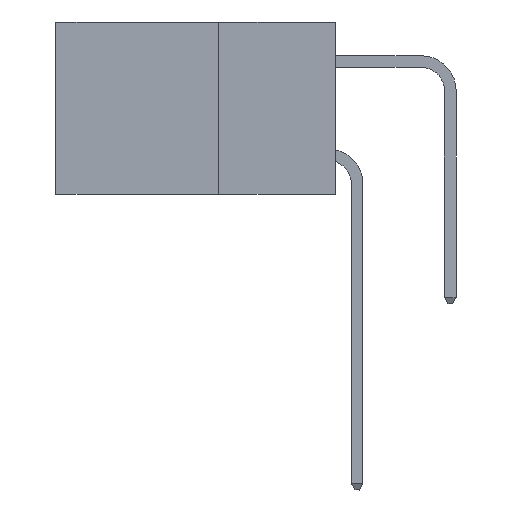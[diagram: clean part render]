
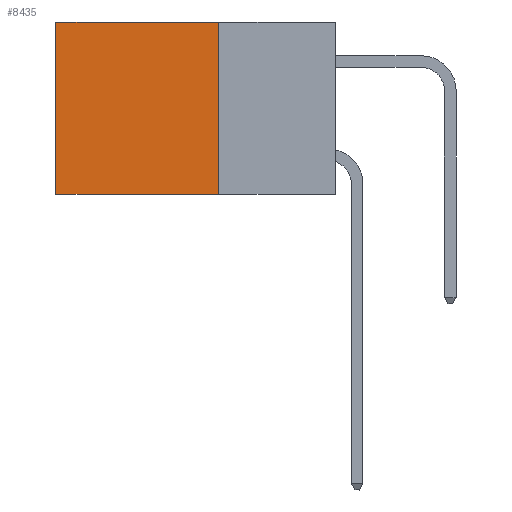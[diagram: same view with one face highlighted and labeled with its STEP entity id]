
A CAD part, left-side view. The second image highlights one B-rep face of the part: STEP entity #8435.
In plain terms, the highlighted planar face has unit normal (-1, 0, 0).
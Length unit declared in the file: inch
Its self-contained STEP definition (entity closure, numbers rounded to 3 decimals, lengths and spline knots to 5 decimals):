
#337 = CARTESIAN_POINT ( 'NONE',  ( 0.2875, 0.25, 0. ) ) ;
#356 = LINE ( 'NONE', #12097, #19102 ) ;
#417 = VECTOR ( 'NONE', #13929, 39.37008 ) ;
#783 = CARTESIAN_POINT ( 'NONE',  ( 0.2875, 0.6, -0.37 ) ) ;
#3746 = AXIS2_PLACEMENT_3D ( 'NONE', #16831, #9396, #17140 ) ;
#4080 = DIRECTION ( 'NONE',  ( 0., 0., -1. ) ) ;
#4876 = LINE ( 'NONE', #337, #417 ) ;
#5610 = CARTESIAN_POINT ( 'NONE',  ( 0.2875, 0.6, 0. ) ) ;
#6252 = VECTOR ( 'NONE', #9681, 39.37008 ) ;
#6415 = EDGE_CURVE ( 'NONE', #13733, #8598, #4876, .T. ) ;
#6735 = CARTESIAN_POINT ( 'NONE',  ( 0.2875, 0.25, -0.37 ) ) ;
#7536 = EDGE_CURVE ( 'NONE', #13733, #16160, #356, .T. ) ;
#7782 = ORIENTED_EDGE ( 'NONE', *, *, #8490, .F. ) ;
#8435 = ADVANCED_FACE ( 'NONE', ( #18331 ), #10872, .F. ) ;
#8490 = EDGE_CURVE ( 'NONE', #8598, #8946, #9591, .T. ) ;
#8598 = VERTEX_POINT ( 'NONE', #9781 ) ;
#8946 = VERTEX_POINT ( 'NONE', #783 ) ;
#9396 = DIRECTION ( 'NONE',  ( 1., 0., 0. ) ) ;
#9421 = CARTESIAN_POINT ( 'NONE',  ( 0.2875, 0.25, 0. ) ) ;
#9540 = DIRECTION ( 'NONE',  ( 0., 1., 0. ) ) ;
#9591 = LINE ( 'NONE', #6735, #6252 ) ;
#9681 = DIRECTION ( 'NONE',  ( 0., 1., 0. ) ) ;
#9781 = CARTESIAN_POINT ( 'NONE',  ( 0.2875, 0.25, -0.37 ) ) ;
#10872 = PLANE ( 'NONE',  #3746 ) ;
#11330 = ORIENTED_EDGE ( 'NONE', *, *, #6415, .F. ) ;
#12097 = CARTESIAN_POINT ( 'NONE',  ( 0.2875, 0.25, 0. ) ) ;
#13052 = ORIENTED_EDGE ( 'NONE', *, *, #7536, .T. ) ;
#13733 = VERTEX_POINT ( 'NONE', #9421 ) ;
#13863 = EDGE_CURVE ( 'NONE', #16160, #8946, #14322, .T. ) ;
#13929 = DIRECTION ( 'NONE',  ( 0., 0., -1. ) ) ;
#14322 = LINE ( 'NONE', #17553, #17335 ) ;
#14951 = EDGE_LOOP ( 'NONE', ( #16659, #7782, #11330, #13052 ) ) ;
#16160 = VERTEX_POINT ( 'NONE', #5610 ) ;
#16659 = ORIENTED_EDGE ( 'NONE', *, *, #13863, .T. ) ;
#16831 = CARTESIAN_POINT ( 'NONE',  ( 0.2875, 0.25, 0. ) ) ;
#17140 = DIRECTION ( 'NONE',  ( 0., 0., -1. ) ) ;
#17335 = VECTOR ( 'NONE', #4080, 39.37008 ) ;
#17553 = CARTESIAN_POINT ( 'NONE',  ( 0.2875, 0.6, 0. ) ) ;
#18331 = FACE_OUTER_BOUND ( 'NONE', #14951, .T. ) ;
#19102 = VECTOR ( 'NONE', #9540, 39.37008 ) ;
